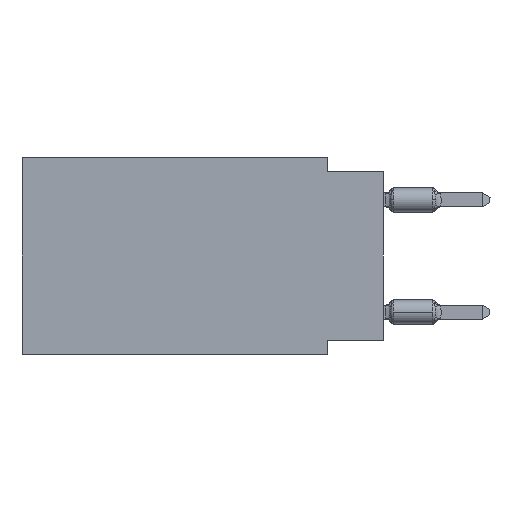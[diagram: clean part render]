
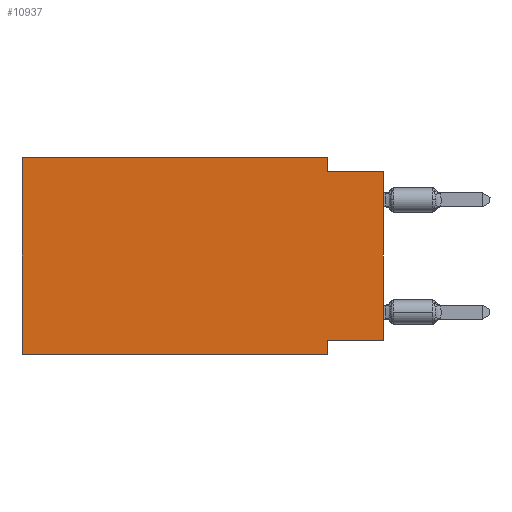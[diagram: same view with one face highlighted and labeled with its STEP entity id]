
A CAD part, left-side view. The second image highlights one B-rep face of the part: STEP entity #10937.
In plain terms, the highlighted planar face has unit normal (-1, 0, 0).
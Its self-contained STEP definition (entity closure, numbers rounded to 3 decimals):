
#844 = CARTESIAN_POINT ( 'NONE',  ( 0., 16.383, 0. ) ) ;
#1056 = CARTESIAN_POINT ( 'NONE',  ( 0., 0., -8.255 ) ) ;
#1354 = DIRECTION ( 'NONE',  ( 0., -1., 0. ) ) ;
#1644 = LINE ( 'NONE', #28588, #23737 ) ;
#1757 = CARTESIAN_POINT ( 'NONE',  ( 0., 16.383, 0. ) ) ;
#1778 = CARTESIAN_POINT ( 'NONE',  ( 0., 16.383, -8.89 ) ) ;
#1842 = VERTEX_POINT ( 'NONE', #7724 ) ;
#2540 = EDGE_CURVE ( 'NONE', #1842, #15303, #8677, .T. ) ;
#3182 = PLANE ( 'NONE',  #17485 ) ;
#4083 = DIRECTION ( 'NONE',  ( 0., 0., -1. ) ) ;
#4478 = CARTESIAN_POINT ( 'NONE',  ( 0., 2.54, -8.255 ) ) ;
#4883 = EDGE_CURVE ( 'NONE', #4967, #26119, #10321, .T. ) ;
#4967 = VERTEX_POINT ( 'NONE', #28589 ) ;
#5230 = DIRECTION ( 'NONE',  ( 0., 0., -1. ) ) ;
#5568 = VECTOR ( 'NONE', #28693, 1000. ) ;
#5605 = CARTESIAN_POINT ( 'NONE',  ( 0., 0., -0.635 ) ) ;
#5867 = LINE ( 'NONE', #19762, #5568 ) ;
#6560 = ORIENTED_EDGE ( 'NONE', *, *, #15318, .F. ) ;
#7724 = CARTESIAN_POINT ( 'NONE',  ( 0., 16.383, -8.89 ) ) ;
#7818 = LINE ( 'NONE', #5605, #20972 ) ;
#8525 = CARTESIAN_POINT ( 'NONE',  ( 0., 2.54, 0. ) ) ;
#8673 = ORIENTED_EDGE ( 'NONE', *, *, #2540, .F. ) ;
#8677 = LINE ( 'NONE', #9269, #22710 ) ;
#9269 = CARTESIAN_POINT ( 'NONE',  ( 0., 16.383, 0. ) ) ;
#9984 = ORIENTED_EDGE ( 'NONE', *, *, #19526, .F. ) ;
#10321 = LINE ( 'NONE', #8525, #17466 ) ;
#10606 = DIRECTION ( 'NONE',  ( 0., 0., -1. ) ) ;
#10620 = ORIENTED_EDGE ( 'NONE', *, *, #4883, .F. ) ;
#10730 = DIRECTION ( 'NONE',  ( 0., -1., 0. ) ) ;
#10937 = ADVANCED_FACE ( 'NONE', ( #18997 ), #3182, .F. ) ;
#11888 = VECTOR ( 'NONE', #10730, 1000. ) ;
#12984 = CARTESIAN_POINT ( 'NONE',  ( 0., 2.54, -0.635 ) ) ;
#13223 = EDGE_CURVE ( 'NONE', #14703, #25128, #13232, .T. ) ;
#13232 = LINE ( 'NONE', #28610, #15298 ) ;
#14583 = VECTOR ( 'NONE', #4083, 1000. ) ;
#14690 = EDGE_CURVE ( 'NONE', #26119, #25128, #7818, .T. ) ;
#14703 = VERTEX_POINT ( 'NONE', #1056 ) ;
#15298 = VECTOR ( 'NONE', #24220, 1000. ) ;
#15303 = VERTEX_POINT ( 'NONE', #1757 ) ;
#15318 = EDGE_CURVE ( 'NONE', #15303, #4967, #5867, .T. ) ;
#17163 = CARTESIAN_POINT ( 'NONE',  ( 0., 0., -0.635 ) ) ;
#17466 = VECTOR ( 'NONE', #10606, 1000. ) ;
#17485 = AXIS2_PLACEMENT_3D ( 'NONE', #844, #27785, #5230 ) ;
#17597 = VERTEX_POINT ( 'NONE', #4478 ) ;
#18352 = ORIENTED_EDGE ( 'NONE', *, *, #13223, .T. ) ;
#18997 = FACE_OUTER_BOUND ( 'NONE', #24351, .T. ) ;
#19526 = EDGE_CURVE ( 'NONE', #14703, #17597, #1644, .T. ) ;
#19611 = LINE ( 'NONE', #28538, #14583 ) ;
#19762 = CARTESIAN_POINT ( 'NONE',  ( 0., 16.383, 0. ) ) ;
#20972 = VECTOR ( 'NONE', #1354, 1000. ) ;
#21299 = ORIENTED_EDGE ( 'NONE', *, *, #26976, .F. ) ;
#21854 = LINE ( 'NONE', #1778, #11888 ) ;
#22710 = VECTOR ( 'NONE', #24639, 1000. ) ;
#23672 = ORIENTED_EDGE ( 'NONE', *, *, #14690, .F. ) ;
#23737 = VECTOR ( 'NONE', #23909, 1000. ) ;
#23909 = DIRECTION ( 'NONE',  ( 0., 1., 0. ) ) ;
#24220 = DIRECTION ( 'NONE',  ( 0., 0., 1. ) ) ;
#24351 = EDGE_LOOP ( 'NONE', ( #18352, #23672, #10620, #6560, #8673, #24983, #21299, #9984 ) ) ;
#24639 = DIRECTION ( 'NONE',  ( 0., 0., 1. ) ) ;
#24983 = ORIENTED_EDGE ( 'NONE', *, *, #28935, .T. ) ;
#25128 = VERTEX_POINT ( 'NONE', #17163 ) ;
#26119 = VERTEX_POINT ( 'NONE', #12984 ) ;
#26976 = EDGE_CURVE ( 'NONE', #17597, #27349, #19611, .T. ) ;
#27349 = VERTEX_POINT ( 'NONE', #28936 ) ;
#27785 = DIRECTION ( 'NONE',  ( 1., 0., 0. ) ) ;
#28538 = CARTESIAN_POINT ( 'NONE',  ( 0., 2.54, -8.89 ) ) ;
#28588 = CARTESIAN_POINT ( 'NONE',  ( 0., 0., -8.255 ) ) ;
#28589 = CARTESIAN_POINT ( 'NONE',  ( 0., 2.54, 0. ) ) ;
#28610 = CARTESIAN_POINT ( 'NONE',  ( 0., 0., 0. ) ) ;
#28693 = DIRECTION ( 'NONE',  ( 0., -1., 0. ) ) ;
#28935 = EDGE_CURVE ( 'NONE', #1842, #27349, #21854, .T. ) ;
#28936 = CARTESIAN_POINT ( 'NONE',  ( 0., 2.54, -8.89 ) ) ;
